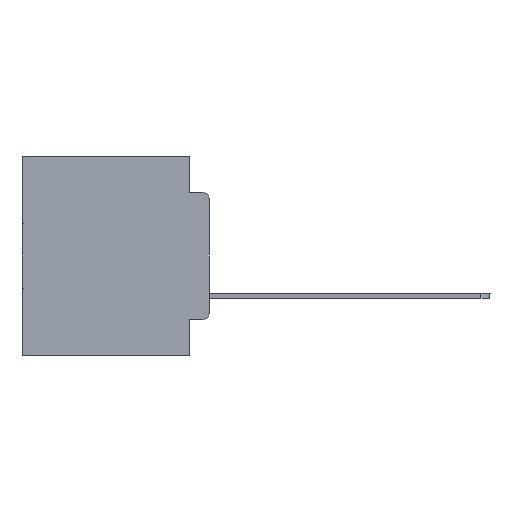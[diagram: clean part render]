
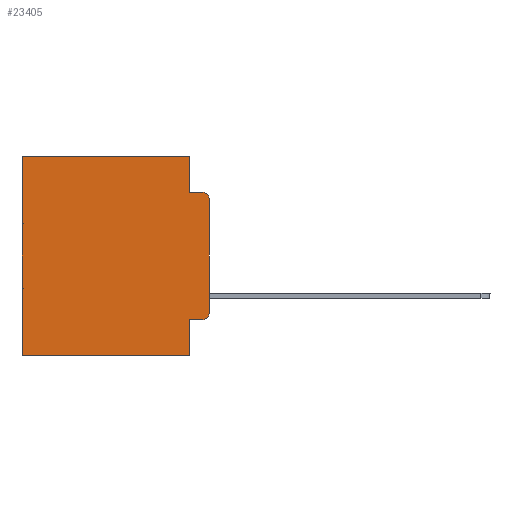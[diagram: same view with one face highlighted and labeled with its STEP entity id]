
A CAD part, left-side view. The second image highlights one B-rep face of the part: STEP entity #23405.
In plain terms, the highlighted planar face has unit normal (-1, 0, 0).
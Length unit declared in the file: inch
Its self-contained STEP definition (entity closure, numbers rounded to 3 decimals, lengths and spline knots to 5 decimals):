
#14 = VERTEX_POINT ( 'NONE', #8181 ) ;
#237 = CARTESIAN_POINT ( 'NONE',  ( 0.298, 0.051, -0.0885 ) ) ;
#558 = AXIS2_PLACEMENT_3D ( 'NONE', #29911, #10269, #20351 ) ;
#763 = LINE ( 'NONE', #20862, #20997 ) ;
#971 = DIRECTION ( 'NONE',  ( -1., 0., 0. ) ) ;
#1007 = VERTEX_POINT ( 'NONE', #22942 ) ;
#1124 = ORIENTED_EDGE ( 'NONE', *, *, #8964, .T. ) ;
#2958 = VERTEX_POINT ( 'NONE', #29287 ) ;
#3027 = DIRECTION ( 'NONE',  ( 0., 0., -1. ) ) ;
#3119 = CIRCLE ( 'NONE', #12022, 0.02 ) ;
#3547 = VERTEX_POINT ( 'NONE', #14599 ) ;
#3681 = LINE ( 'NONE', #13616, #30747 ) ;
#3733 = LINE ( 'NONE', #12950, #4911 ) ;
#3814 = EDGE_CURVE ( 'NONE', #8682, #3967, #763, .T. ) ;
#3967 = VERTEX_POINT ( 'NONE', #22740 ) ;
#4669 = CARTESIAN_POINT ( 'NONE',  ( 0.298, 0.473, 0. ) ) ;
#4911 = VECTOR ( 'NONE', #3027, 39.37008 ) ;
#5276 = VERTEX_POINT ( 'NONE', #4669 ) ;
#5877 = LINE ( 'NONE', #23255, #23352 ) ;
#5979 = CARTESIAN_POINT ( 'NONE',  ( 0.298, 0.02, -0.3915 ) ) ;
#5984 = CARTESIAN_POINT ( 'NONE',  ( 0.298, 0.02, -0.1085 ) ) ;
#6437 = DIRECTION ( 'NONE',  ( -1., 0., 0. ) ) ;
#6489 = ORIENTED_EDGE ( 'NONE', *, *, #22495, .F. ) ;
#7574 = PLANE ( 'NONE',  #558 ) ;
#8181 = CARTESIAN_POINT ( 'NONE',  ( 0.298, 0.473, -0.5 ) ) ;
#8682 = VERTEX_POINT ( 'NONE', #12653 ) ;
#8964 = EDGE_CURVE ( 'NONE', #25316, #5276, #31521, .T. ) ;
#9174 = ORIENTED_EDGE ( 'NONE', *, *, #10435, .T. ) ;
#9337 = CARTESIAN_POINT ( 'NONE',  ( 0.298, 0.02, -0.4115 ) ) ;
#9424 = VECTOR ( 'NONE', #10652, 39.37008 ) ;
#9724 = ORIENTED_EDGE ( 'NONE', *, *, #22248, .T. ) ;
#10269 = DIRECTION ( 'NONE',  ( 1., 0., 0. ) ) ;
#10435 = EDGE_CURVE ( 'NONE', #12399, #21505, #3119, .T. ) ;
#10652 = DIRECTION ( 'NONE',  ( 0., 0., -1. ) ) ;
#10852 = DIRECTION ( 'NONE',  ( 0., 0., -1. ) ) ;
#10980 = DIRECTION ( 'NONE',  ( 0., 0., -1. ) ) ;
#12022 = AXIS2_PLACEMENT_3D ( 'NONE', #5979, #6437, #23452 ) ;
#12399 = VERTEX_POINT ( 'NONE', #9337 ) ;
#12637 = CARTESIAN_POINT ( 'NONE',  ( 0.298, 0.051, 0. ) ) ;
#12653 = CARTESIAN_POINT ( 'NONE',  ( 0.298, 0.051, -0.4115 ) ) ;
#12950 = CARTESIAN_POINT ( 'NONE',  ( 0.298, 0.473, 0. ) ) ;
#13616 = CARTESIAN_POINT ( 'NONE',  ( 0.298, 0.051, -0.4115 ) ) ;
#13747 = FACE_OUTER_BOUND ( 'NONE', #28028, .T. ) ;
#14599 = CARTESIAN_POINT ( 'NONE',  ( 0.298, 0., -0.1085 ) ) ;
#15149 = VECTOR ( 'NONE', #23101, 39.37008 ) ;
#15496 = CARTESIAN_POINT ( 'NONE',  ( 0.298, 0.051, 0. ) ) ;
#15717 = LINE ( 'NONE', #237, #25016 ) ;
#16389 = LINE ( 'NONE', #15496, #9424 ) ;
#16537 = DIRECTION ( 'NONE',  ( 0., 1., 0. ) ) ;
#17602 = DIRECTION ( 'NONE',  ( 0., -1., 0. ) ) ;
#17798 = CARTESIAN_POINT ( 'NONE',  ( 0.298, 0., -0.5 ) ) ;
#18357 = EDGE_CURVE ( 'NONE', #25316, #2958, #16389, .T. ) ;
#19013 = EDGE_CURVE ( 'NONE', #3967, #14, #20975, .T. ) ;
#19243 = ORIENTED_EDGE ( 'NONE', *, *, #24103, .T. ) ;
#19585 = CIRCLE ( 'NONE', #20408, 0.02 ) ;
#20351 = DIRECTION ( 'NONE',  ( 0., 0., -1. ) ) ;
#20408 = AXIS2_PLACEMENT_3D ( 'NONE', #5984, #971, #25566 ) ;
#20862 = CARTESIAN_POINT ( 'NONE',  ( 0.298, 0.051, 0. ) ) ;
#20975 = LINE ( 'NONE', #17798, #15149 ) ;
#20997 = VECTOR ( 'NONE', #10852, 39.37008 ) ;
#21505 = VERTEX_POINT ( 'NONE', #30232 ) ;
#22248 = EDGE_CURVE ( 'NONE', #8682, #12399, #3681, .T. ) ;
#22495 = EDGE_CURVE ( 'NONE', #2958, #1007, #15717, .T. ) ;
#22740 = CARTESIAN_POINT ( 'NONE',  ( 0.298, 0.051, -0.5 ) ) ;
#22942 = CARTESIAN_POINT ( 'NONE',  ( 0.298, 0.02, -0.0885 ) ) ;
#23101 = DIRECTION ( 'NONE',  ( 0., 1., 0. ) ) ;
#23255 = CARTESIAN_POINT ( 'NONE',  ( 0.298, 0., 0. ) ) ;
#23352 = VECTOR ( 'NONE', #10980, 39.37008 ) ;
#23405 = ADVANCED_FACE ( 'NONE', ( #13747 ), #7574, .F. ) ;
#23452 = DIRECTION ( 'NONE',  ( 0., 0., -1. ) ) ;
#24103 = EDGE_CURVE ( 'NONE', #5276, #14, #3733, .T. ) ;
#24995 = ORIENTED_EDGE ( 'NONE', *, *, #19013, .F. ) ;
#25016 = VECTOR ( 'NONE', #17602, 39.37008 ) ;
#25316 = VERTEX_POINT ( 'NONE', #12637 ) ;
#25486 = ORIENTED_EDGE ( 'NONE', *, *, #30907, .F. ) ;
#25566 = DIRECTION ( 'NONE',  ( 0., 0., -1. ) ) ;
#25587 = DIRECTION ( 'NONE',  ( 0., -1., 0. ) ) ;
#25741 = VECTOR ( 'NONE', #16537, 39.37008 ) ;
#26376 = EDGE_CURVE ( 'NONE', #3547, #1007, #19585, .T. ) ;
#26768 = ORIENTED_EDGE ( 'NONE', *, *, #3814, .F. ) ;
#27124 = ORIENTED_EDGE ( 'NONE', *, *, #18357, .F. ) ;
#27455 = ORIENTED_EDGE ( 'NONE', *, *, #26376, .T. ) ;
#28028 = EDGE_LOOP ( 'NONE', ( #25486, #27455, #6489, #27124, #1124, #19243, #24995, #26768, #9724, #9174 ) ) ;
#28791 = CARTESIAN_POINT ( 'NONE',  ( 0.298, 0., 0. ) ) ;
#29287 = CARTESIAN_POINT ( 'NONE',  ( 0.298, 0.051, -0.0885 ) ) ;
#29911 = CARTESIAN_POINT ( 'NONE',  ( 0.298, 0., 0. ) ) ;
#30232 = CARTESIAN_POINT ( 'NONE',  ( 0.298, 0., -0.3915 ) ) ;
#30747 = VECTOR ( 'NONE', #25587, 39.37008 ) ;
#30907 = EDGE_CURVE ( 'NONE', #3547, #21505, #5877, .T. ) ;
#31521 = LINE ( 'NONE', #28791, #25741 ) ;
